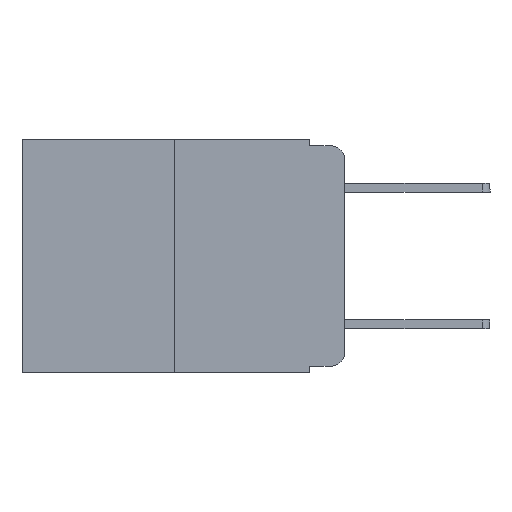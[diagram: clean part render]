
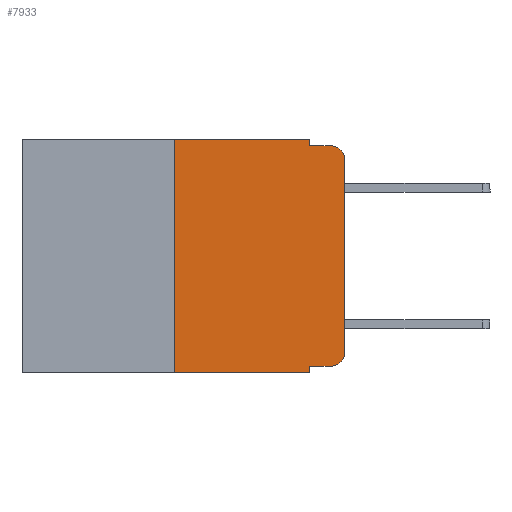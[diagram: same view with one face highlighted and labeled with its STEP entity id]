
A CAD part, left-side view. The second image highlights one B-rep face of the part: STEP entity #7933.
In plain terms, the highlighted planar face has unit normal (-1, 0, 0).
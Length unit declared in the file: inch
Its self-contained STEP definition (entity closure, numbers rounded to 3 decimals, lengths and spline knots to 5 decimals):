
#583 = CARTESIAN_POINT ( 'NONE',  ( 0., 0.25, 0. ) ) ;
#676 = CIRCLE ( 'NONE', #9593, 0.02 ) ;
#1042 = ORIENTED_EDGE ( 'NONE', *, *, #15560, .F. ) ;
#1617 = CIRCLE ( 'NONE', #5872, 0.02 ) ;
#2472 = ORIENTED_EDGE ( 'NONE', *, *, #8463, .F. ) ;
#2548 = ORIENTED_EDGE ( 'NONE', *, *, #20470, .T. ) ;
#3106 = FACE_OUTER_BOUND ( 'NONE', #4714, .T. ) ;
#3120 = CARTESIAN_POINT ( 'NONE',  ( 0., 0.473, -0.343 ) ) ;
#3362 = DIRECTION ( 'NONE',  ( 1., 0., 0. ) ) ;
#3570 = EDGE_CURVE ( 'NONE', #13999, #15353, #676, .T. ) ;
#3938 = DIRECTION ( 'NONE',  ( 0., -1., 0. ) ) ;
#3985 = CARTESIAN_POINT ( 'NONE',  ( 0., 0.051, -0.333 ) ) ;
#4210 = VECTOR ( 'NONE', #25066, 39.37008 ) ;
#4355 = CARTESIAN_POINT ( 'NONE',  ( 0., 0.051, -0.01 ) ) ;
#4714 = EDGE_LOOP ( 'NONE', ( #11789, #4948, #14590, #20135, #2472, #1042, #2548, #24779, #15851, #10229 ) ) ;
#4948 = ORIENTED_EDGE ( 'NONE', *, *, #10775, .T. ) ;
#5330 = VECTOR ( 'NONE', #20707, 39.37008 ) ;
#5872 = AXIS2_PLACEMENT_3D ( 'NONE', #13712, #13598, #9479 ) ;
#6062 = DIRECTION ( 'NONE',  ( 0., -1., 0. ) ) ;
#6108 = DIRECTION ( 'NONE',  ( -1., 0., 0. ) ) ;
#6122 = DIRECTION ( 'NONE',  ( 0., 0., 1. ) ) ;
#6596 = VERTEX_POINT ( 'NONE', #10813 ) ;
#6615 = CARTESIAN_POINT ( 'NONE',  ( 0., 0.473, 0. ) ) ;
#6700 = DIRECTION ( 'NONE',  ( 0., 0., 1. ) ) ;
#6954 = CARTESIAN_POINT ( 'NONE',  ( 0., 0., 0. ) ) ;
#7223 = PLANE ( 'NONE',  #23549 ) ;
#7789 = VERTEX_POINT ( 'NONE', #10818 ) ;
#7933 = ADVANCED_FACE ( 'NONE', ( #3106 ), #7223, .F. ) ;
#8463 = EDGE_CURVE ( 'NONE', #18475, #11795, #17116, .T. ) ;
#9338 = CARTESIAN_POINT ( 'NONE',  ( 0., 0.02, -0.333 ) ) ;
#9479 = DIRECTION ( 'NONE',  ( 0., 0., -1. ) ) ;
#9593 = AXIS2_PLACEMENT_3D ( 'NONE', #26193, #6108, #14213 ) ;
#10229 = ORIENTED_EDGE ( 'NONE', *, *, #3570, .T. ) ;
#10775 = EDGE_CURVE ( 'NONE', #15643, #20009, #1617, .T. ) ;
#10813 = CARTESIAN_POINT ( 'NONE',  ( 0., 0.25, -0.343 ) ) ;
#10818 = CARTESIAN_POINT ( 'NONE',  ( 0., 0.051, -0.343 ) ) ;
#11356 = DIRECTION ( 'NONE',  ( 0., 0., -1. ) ) ;
#11789 = ORIENTED_EDGE ( 'NONE', *, *, #18505, .T. ) ;
#11795 = VERTEX_POINT ( 'NONE', #14157 ) ;
#12656 = VECTOR ( 'NONE', #6062, 39.37008 ) ;
#12860 = VERTEX_POINT ( 'NONE', #4355 ) ;
#13085 = LINE ( 'NONE', #3120, #4210 ) ;
#13598 = DIRECTION ( 'NONE',  ( -1., 0., 0. ) ) ;
#13712 = CARTESIAN_POINT ( 'NONE',  ( 0., 0.02, -0.03 ) ) ;
#13893 = LINE ( 'NONE', #18007, #25010 ) ;
#13999 = VERTEX_POINT ( 'NONE', #9338 ) ;
#14157 = CARTESIAN_POINT ( 'NONE',  ( 0., 0.051, 0. ) ) ;
#14164 = CARTESIAN_POINT ( 'NONE',  ( 0., 0.051, -0.333 ) ) ;
#14213 = DIRECTION ( 'NONE',  ( 0., 0., -1. ) ) ;
#14489 = EDGE_CURVE ( 'NONE', #17907, #13999, #15885, .T. ) ;
#14590 = ORIENTED_EDGE ( 'NONE', *, *, #20071, .F. ) ;
#15353 = VERTEX_POINT ( 'NONE', #19285 ) ;
#15450 = DIRECTION ( 'NONE',  ( 0., 0., -1. ) ) ;
#15459 = CARTESIAN_POINT ( 'NONE',  ( 0., 0.051, 0. ) ) ;
#15560 = EDGE_CURVE ( 'NONE', #6596, #18475, #24339, .T. ) ;
#15643 = VERTEX_POINT ( 'NONE', #18232 ) ;
#15851 = ORIENTED_EDGE ( 'NONE', *, *, #14489, .T. ) ;
#15885 = LINE ( 'NONE', #14164, #12656 ) ;
#16233 = CARTESIAN_POINT ( 'NONE',  ( 0., 0.25, 0. ) ) ;
#17071 = LINE ( 'NONE', #6954, #18629 ) ;
#17116 = LINE ( 'NONE', #6615, #5330 ) ;
#17373 = CARTESIAN_POINT ( 'NONE',  ( 0., 0.02, -0.01 ) ) ;
#17582 = LINE ( 'NONE', #15459, #23398 ) ;
#17675 = LINE ( 'NONE', #19668, #19476 ) ;
#17907 = VERTEX_POINT ( 'NONE', #3985 ) ;
#18007 = CARTESIAN_POINT ( 'NONE',  ( 0., 0.051, -0.01 ) ) ;
#18232 = CARTESIAN_POINT ( 'NONE',  ( 0., 0., -0.03 ) ) ;
#18475 = VERTEX_POINT ( 'NONE', #583 ) ;
#18505 = EDGE_CURVE ( 'NONE', #15353, #15643, #17071, .T. ) ;
#18629 = VECTOR ( 'NONE', #6700, 39.37008 ) ;
#19018 = EDGE_CURVE ( 'NONE', #11795, #12860, #17675, .T. ) ;
#19285 = CARTESIAN_POINT ( 'NONE',  ( 0., 0., -0.313 ) ) ;
#19476 = VECTOR ( 'NONE', #23535, 39.37008 ) ;
#19668 = CARTESIAN_POINT ( 'NONE',  ( 0., 0.051, 0. ) ) ;
#20009 = VERTEX_POINT ( 'NONE', #17373 ) ;
#20071 = EDGE_CURVE ( 'NONE', #12860, #20009, #13893, .T. ) ;
#20135 = ORIENTED_EDGE ( 'NONE', *, *, #19018, .F. ) ;
#20470 = EDGE_CURVE ( 'NONE', #6596, #7789, #13085, .T. ) ;
#20707 = DIRECTION ( 'NONE',  ( 0., -1., 0. ) ) ;
#21562 = CARTESIAN_POINT ( 'NONE',  ( 0., 0.473, 0. ) ) ;
#22864 = EDGE_CURVE ( 'NONE', #17907, #7789, #17582, .T. ) ;
#23398 = VECTOR ( 'NONE', #11356, 39.37008 ) ;
#23535 = DIRECTION ( 'NONE',  ( 0., 0., -1. ) ) ;
#23549 = AXIS2_PLACEMENT_3D ( 'NONE', #21562, #3362, #15450 ) ;
#24339 = LINE ( 'NONE', #16233, #25437 ) ;
#24779 = ORIENTED_EDGE ( 'NONE', *, *, #22864, .F. ) ;
#25010 = VECTOR ( 'NONE', #3938, 39.37008 ) ;
#25066 = DIRECTION ( 'NONE',  ( 0., -1., 0. ) ) ;
#25437 = VECTOR ( 'NONE', #6122, 39.37008 ) ;
#26193 = CARTESIAN_POINT ( 'NONE',  ( 0., 0.02, -0.313 ) ) ;
